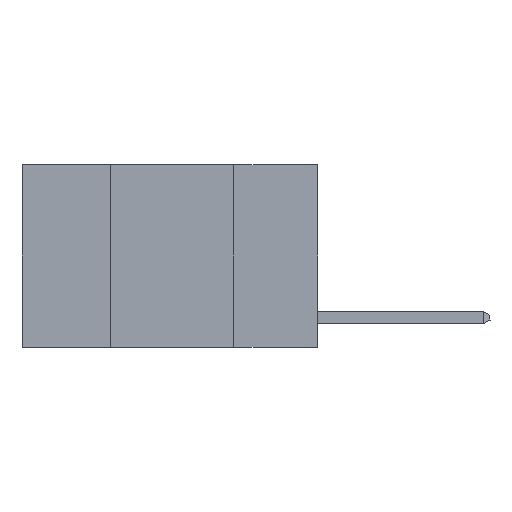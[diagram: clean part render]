
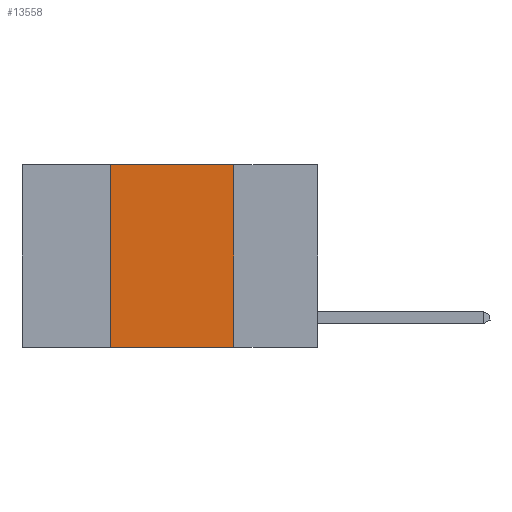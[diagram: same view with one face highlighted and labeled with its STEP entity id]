
A CAD part, left-side view. The second image highlights one B-rep face of the part: STEP entity #13558.
In plain terms, the highlighted planar face has unit normal (-1, 0, 0).
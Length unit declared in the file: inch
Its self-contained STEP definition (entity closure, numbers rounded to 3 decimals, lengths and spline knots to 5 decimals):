
#515 = LINE ( 'NONE', #3162, #4105 ) ;
#536 = EDGE_CURVE ( 'NONE', #11100, #1680, #515, .T. ) ;
#1083 = ORIENTED_EDGE ( 'NONE', *, *, #3227, .F. ) ;
#1365 = CARTESIAN_POINT ( 'NONE',  ( 0., 0.17, 0. ) ) ;
#1406 = FACE_OUTER_BOUND ( 'NONE', #11848, .T. ) ;
#1425 = ORIENTED_EDGE ( 'NONE', *, *, #3466, .F. ) ;
#1680 = VERTEX_POINT ( 'NONE', #3729 ) ;
#2464 = ORIENTED_EDGE ( 'NONE', *, *, #536, .T. ) ;
#2966 = DIRECTION ( 'NONE',  ( 0., 0., -1. ) ) ;
#3038 = DIRECTION ( 'NONE',  ( 0., -1., 0. ) ) ;
#3162 = CARTESIAN_POINT ( 'NONE',  ( 0., 0.6, -0.37 ) ) ;
#3227 = EDGE_CURVE ( 'NONE', #11100, #10621, #14041, .T. ) ;
#3466 = EDGE_CURVE ( 'NONE', #6202, #1680, #10627, .T. ) ;
#3729 = CARTESIAN_POINT ( 'NONE',  ( 0., 0.17, -0.37 ) ) ;
#4105 = VECTOR ( 'NONE', #3038, 39.37008 ) ;
#4459 = CARTESIAN_POINT ( 'NONE',  ( 0., 0.42, -0.37 ) ) ;
#4645 = ORIENTED_EDGE ( 'NONE', *, *, #12886, .F. ) ;
#5060 = VECTOR ( 'NONE', #6364, 39.37008 ) ;
#5601 = DIRECTION ( 'NONE',  ( 0., -1., 0. ) ) ;
#5683 = DIRECTION ( 'NONE',  ( 0., 0., -1. ) ) ;
#6202 = VERTEX_POINT ( 'NONE', #7637 ) ;
#6364 = DIRECTION ( 'NONE',  ( 0., 0., 1. ) ) ;
#6882 = CARTESIAN_POINT ( 'NONE',  ( 0., 0.42, 0. ) ) ;
#7151 = VECTOR ( 'NONE', #5601, 39.37008 ) ;
#7637 = CARTESIAN_POINT ( 'NONE',  ( 0., 0.17, 0. ) ) ;
#8302 = PLANE ( 'NONE',  #10676 ) ;
#8486 = CARTESIAN_POINT ( 'NONE',  ( 0., 0.42, 0. ) ) ;
#8758 = CARTESIAN_POINT ( 'NONE',  ( 0., 0.6, 0. ) ) ;
#9390 = DIRECTION ( 'NONE',  ( 1., 0., 0. ) ) ;
#10032 = LINE ( 'NONE', #8758, #7151 ) ;
#10449 = CARTESIAN_POINT ( 'NONE',  ( 0., 0.6, 0. ) ) ;
#10621 = VERTEX_POINT ( 'NONE', #6882 ) ;
#10627 = LINE ( 'NONE', #1365, #13181 ) ;
#10676 = AXIS2_PLACEMENT_3D ( 'NONE', #10449, #9390, #2966 ) ;
#11100 = VERTEX_POINT ( 'NONE', #4459 ) ;
#11848 = EDGE_LOOP ( 'NONE', ( #1425, #4645, #1083, #2464 ) ) ;
#12886 = EDGE_CURVE ( 'NONE', #10621, #6202, #10032, .T. ) ;
#13181 = VECTOR ( 'NONE', #5683, 39.37008 ) ;
#13558 = ADVANCED_FACE ( 'NONE', ( #1406 ), #8302, .F. ) ;
#14041 = LINE ( 'NONE', #8486, #5060 ) ;
